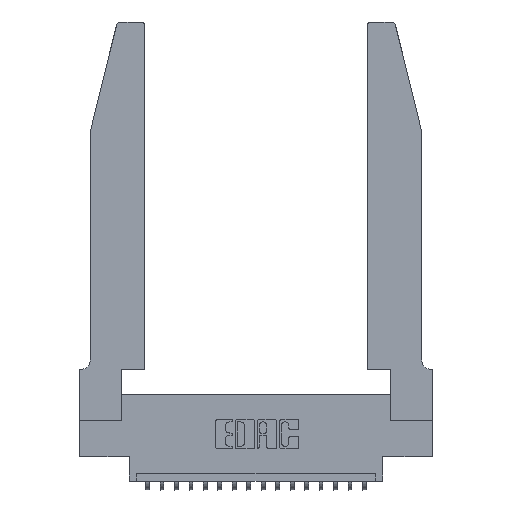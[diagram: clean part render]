
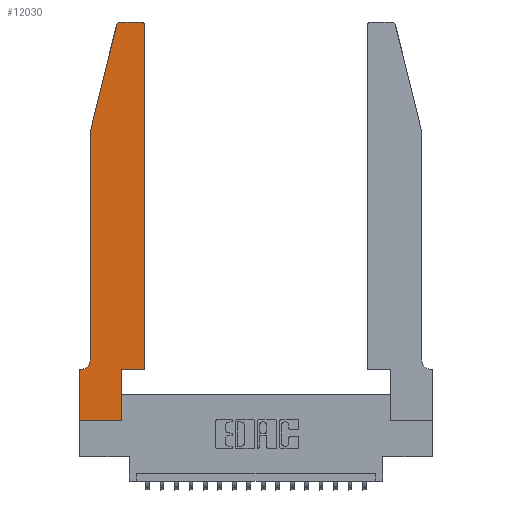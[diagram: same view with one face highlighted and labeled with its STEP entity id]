
A CAD part, top view. The second image highlights one B-rep face of the part: STEP entity #12030.
In plain terms, the highlighted planar face has unit normal (0, 0, 1).
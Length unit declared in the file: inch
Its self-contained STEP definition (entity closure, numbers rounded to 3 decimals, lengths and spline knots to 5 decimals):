
#335 = ORIENTED_EDGE ( 'NONE', *, *, #17758, .T. ) ;
#671 = CARTESIAN_POINT ( 'NONE',  ( 0.4505, 0.35, 0.37 ) ) ;
#752 = DIRECTION ( 'NONE',  ( -1., 0., 0. ) ) ;
#900 = LINE ( 'NONE', #1008, #7341 ) ;
#1008 = CARTESIAN_POINT ( 'NONE',  ( 0.0755, 2., 0.37 ) ) ;
#1051 = EDGE_CURVE ( 'NONE', #2489, #13461, #17104, .T. ) ;
#1260 = CARTESIAN_POINT ( 'NONE',  ( 0., 0., 0.37 ) ) ;
#1562 = CARTESIAN_POINT ( 'NONE',  ( 0.4205, 2.75, 0.37 ) ) ;
#1744 = VECTOR ( 'NONE', #2894, 39.37008 ) ;
#1808 = EDGE_CURVE ( 'NONE', #14776, #14508, #900, .T. ) ;
#2158 = VECTOR ( 'NONE', #16181, 39.37008 ) ;
#2365 = ORIENTED_EDGE ( 'NONE', *, *, #12718, .T. ) ;
#2448 = LINE ( 'NONE', #17380, #15874 ) ;
#2489 = VERTEX_POINT ( 'NONE', #10567 ) ;
#2547 = CARTESIAN_POINT ( 'NONE',  ( 0.4205, 2.72, 0.37 ) ) ;
#2894 = DIRECTION ( 'NONE',  ( 1., 0., 0. ) ) ;
#2943 = ORIENTED_EDGE ( 'NONE', *, *, #3364, .T. ) ;
#3018 = VERTEX_POINT ( 'NONE', #10035 ) ;
#3328 = ORIENTED_EDGE ( 'NONE', *, *, #1051, .T. ) ;
#3364 = EDGE_CURVE ( 'NONE', #17656, #14776, #11972, .T. ) ;
#4020 = DIRECTION ( 'NONE',  ( 0., -1., 0. ) ) ;
#4369 = DIRECTION ( 'NONE',  ( 0., 0., 1. ) ) ;
#4750 = VECTOR ( 'NONE', #9991, 39.37008 ) ;
#4846 = ORIENTED_EDGE ( 'NONE', *, *, #19207, .T. ) ;
#5086 = VERTEX_POINT ( 'NONE', #13763 ) ;
#5102 = VERTEX_POINT ( 'NONE', #20450 ) ;
#5381 = CIRCLE ( 'NONE', #11130, 0.03 ) ;
#5432 = ORIENTED_EDGE ( 'NONE', *, *, #19744, .T. ) ;
#5742 = LINE ( 'NONE', #11330, #4750 ) ;
#5822 = VERTEX_POINT ( 'NONE', #17033 ) ;
#6003 = CARTESIAN_POINT ( 'NONE',  ( 0., 0.35, 0.37 ) ) ;
#6186 = VECTOR ( 'NONE', #7045, 39.37008 ) ;
#6306 = DIRECTION ( 'NONE',  ( 1., 0., 0. ) ) ;
#6958 = FACE_OUTER_BOUND ( 'NONE', #19062, .T. ) ;
#7045 = DIRECTION ( 'NONE',  ( 1., 0., 0. ) ) ;
#7220 = CARTESIAN_POINT ( 'NONE',  ( 0.2865, 0.35, 0.37 ) ) ;
#7341 = VECTOR ( 'NONE', #4020, 39.37008 ) ;
#7568 = EDGE_CURVE ( 'NONE', #14508, #5086, #13845, .T. ) ;
#7577 = DIRECTION ( 'NONE',  ( -0.239, -0.971, 0. ) ) ;
#7634 = DIRECTION ( 'NONE',  ( 1., 0., 0. ) ) ;
#7746 = VECTOR ( 'NONE', #7577, 39.37008 ) ;
#8170 = CIRCLE ( 'NONE', #13994, 0.03 ) ;
#8228 = EDGE_CURVE ( 'NONE', #5102, #3018, #12835, .T. ) ;
#8237 = EDGE_CURVE ( 'NONE', #10074, #17656, #5381, .T. ) ;
#8324 = CARTESIAN_POINT ( 'NONE',  ( 0.284, 2.75, 0.37 ) ) ;
#8708 = CARTESIAN_POINT ( 'NONE',  ( 0.4505, 2.72, 0.37 ) ) ;
#9848 = ORIENTED_EDGE ( 'NONE', *, *, #14498, .T. ) ;
#9989 = DIRECTION ( 'NONE',  ( 0., 0., -1. ) ) ;
#9991 = DIRECTION ( 'NONE',  ( -1., 0., 0. ) ) ;
#9993 = ORIENTED_EDGE ( 'NONE', *, *, #8237, .T. ) ;
#10035 = CARTESIAN_POINT ( 'NONE',  ( 0., 0., 0.37 ) ) ;
#10074 = VERTEX_POINT ( 'NONE', #8324 ) ;
#10260 = CARTESIAN_POINT ( 'NONE',  ( 0.0055, 0.42, 0.37 ) ) ;
#10565 = CARTESIAN_POINT ( 'NONE',  ( 0.25487, 2.72718, 0.37 ) ) ;
#10567 = CARTESIAN_POINT ( 'NONE',  ( 0.2865, 0.35, 0.37 ) ) ;
#11039 = ORIENTED_EDGE ( 'NONE', *, *, #8228, .T. ) ;
#11110 = VECTOR ( 'NONE', #11517, 39.37008 ) ;
#11130 = AXIS2_PLACEMENT_3D ( 'NONE', #12803, #13352, #13279 ) ;
#11330 = CARTESIAN_POINT ( 'NONE',  ( 0.2605, 2.75, 0.37 ) ) ;
#11517 = DIRECTION ( 'NONE',  ( -1., 0., 0. ) ) ;
#11584 = AXIS2_PLACEMENT_3D ( 'NONE', #6003, #4369, #7634 ) ;
#11972 = LINE ( 'NONE', #20061, #7746 ) ;
#12030 = ADVANCED_FACE ( 'NONE', ( #6958 ), #14115, .T. ) ;
#12299 = AXIS2_PLACEMENT_3D ( 'NONE', #10260, #9989, #752 ) ;
#12405 = DIRECTION ( 'NONE',  ( 0., 1., 0. ) ) ;
#12718 = EDGE_CURVE ( 'NONE', #14167, #16358, #8170, .T. ) ;
#12803 = CARTESIAN_POINT ( 'NONE',  ( 0.284, 2.72, 0.37 ) ) ;
#12835 = LINE ( 'NONE', #17576, #2158 ) ;
#13279 = DIRECTION ( 'NONE',  ( 1., 0., 0. ) ) ;
#13352 = DIRECTION ( 'NONE',  ( 0., 0., 1. ) ) ;
#13358 = VECTOR ( 'NONE', #19898, 39.37008 ) ;
#13417 = LINE ( 'NONE', #1260, #1744 ) ;
#13461 = VERTEX_POINT ( 'NONE', #14412 ) ;
#13668 = DIRECTION ( 'NONE',  ( 0., 0., 1. ) ) ;
#13763 = CARTESIAN_POINT ( 'NONE',  ( 0.0055, 0.35, 0.37 ) ) ;
#13845 = CIRCLE ( 'NONE', #12299, 0.07 ) ;
#13994 = AXIS2_PLACEMENT_3D ( 'NONE', #2547, #13668, #6306 ) ;
#14115 = PLANE ( 'NONE',  #11584 ) ;
#14167 = VERTEX_POINT ( 'NONE', #8708 ) ;
#14412 = CARTESIAN_POINT ( 'NONE',  ( 0.4505, 0.35, 0.37 ) ) ;
#14498 = EDGE_CURVE ( 'NONE', #16358, #10074, #5742, .T. ) ;
#14508 = VERTEX_POINT ( 'NONE', #19343 ) ;
#14776 = VERTEX_POINT ( 'NONE', #17000 ) ;
#15147 = ORIENTED_EDGE ( 'NONE', *, *, #7568, .T. ) ;
#15874 = VECTOR ( 'NONE', #12405, 39.37008 ) ;
#16071 = LINE ( 'NONE', #7220, #13358 ) ;
#16181 = DIRECTION ( 'NONE',  ( 0., -1., 0. ) ) ;
#16295 = ORIENTED_EDGE ( 'NONE', *, *, #1808, .T. ) ;
#16358 = VERTEX_POINT ( 'NONE', #1562 ) ;
#16361 = CARTESIAN_POINT ( 'NONE',  ( 0.0755, 0.35, 0.37 ) ) ;
#17000 = CARTESIAN_POINT ( 'NONE',  ( 0.0755, 2., 0.37 ) ) ;
#17033 = CARTESIAN_POINT ( 'NONE',  ( 0.2865, 0., 0.37 ) ) ;
#17104 = LINE ( 'NONE', #671, #6186 ) ;
#17380 = CARTESIAN_POINT ( 'NONE',  ( 0.4505, 0.35, 0.37 ) ) ;
#17576 = CARTESIAN_POINT ( 'NONE',  ( 0., 0., 0.37 ) ) ;
#17656 = VERTEX_POINT ( 'NONE', #10565 ) ;
#17758 = EDGE_CURVE ( 'NONE', #3018, #5822, #13417, .T. ) ;
#18212 = EDGE_CURVE ( 'NONE', #13461, #14167, #2448, .T. ) ;
#18281 = LINE ( 'NONE', #16361, #11110 ) ;
#19062 = EDGE_LOOP ( 'NONE', ( #9848, #9993, #2943, #16295, #15147, #5432, #11039, #335, #4846, #3328, #19746, #2365 ) ) ;
#19207 = EDGE_CURVE ( 'NONE', #5822, #2489, #16071, .T. ) ;
#19343 = CARTESIAN_POINT ( 'NONE',  ( 0.0755, 0.42, 0.37 ) ) ;
#19744 = EDGE_CURVE ( 'NONE', #5086, #5102, #18281, .T. ) ;
#19746 = ORIENTED_EDGE ( 'NONE', *, *, #18212, .T. ) ;
#19898 = DIRECTION ( 'NONE',  ( 0., 1., 0. ) ) ;
#20061 = CARTESIAN_POINT ( 'NONE',  ( 0.0755, 2., 0.37 ) ) ;
#20450 = CARTESIAN_POINT ( 'NONE',  ( 0., 0.35, 0.37 ) ) ;
